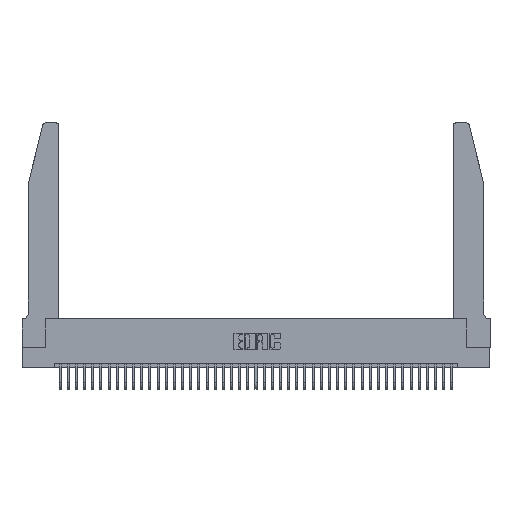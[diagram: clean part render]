
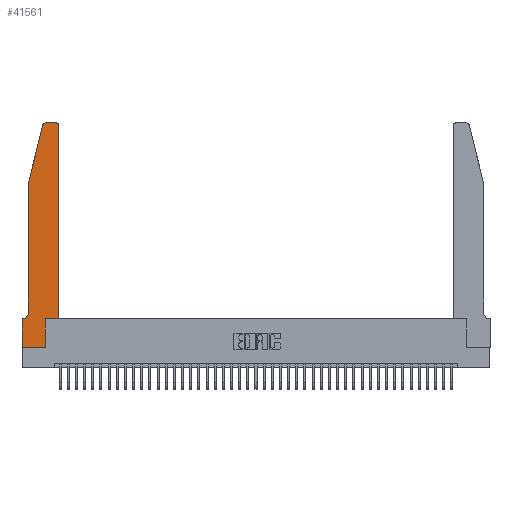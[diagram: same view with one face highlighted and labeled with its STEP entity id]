
A CAD part, top view. The second image highlights one B-rep face of the part: STEP entity #41561.
In plain terms, the highlighted planar face has unit normal (0, 0, 1).
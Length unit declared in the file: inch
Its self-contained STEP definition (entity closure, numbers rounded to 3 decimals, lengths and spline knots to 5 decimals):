
#1439 = CARTESIAN_POINT ( 'NONE',  ( 0.0055, 0.42, 0.37 ) ) ;
#2660 = VERTEX_POINT ( 'NONE', #24972 ) ;
#2988 = LINE ( 'NONE', #31300, #11111 ) ;
#3441 = CIRCLE ( 'NONE', #13869, 0.03 ) ;
#4783 = VERTEX_POINT ( 'NONE', #22623 ) ;
#4931 = DIRECTION ( 'NONE',  ( -1., 0., 0. ) ) ;
#5466 = DIRECTION ( 'NONE',  ( 1., 0., 0. ) ) ;
#5712 = VERTEX_POINT ( 'NONE', #22765 ) ;
#5819 = DIRECTION ( 'NONE',  ( -1., 0., 0. ) ) ;
#6083 = EDGE_CURVE ( 'NONE', #2660, #15268, #40736, .T. ) ;
#6863 = CARTESIAN_POINT ( 'NONE',  ( 0.0755, 0.42, 0.37 ) ) ;
#6955 = EDGE_CURVE ( 'NONE', #35982, #40524, #16182, .T. ) ;
#7196 = EDGE_LOOP ( 'NONE', ( #37225, #29866, #19095, #36758, #37483, #36531, #28214, #31045, #24178, #24218, #27506, #36055 ) ) ;
#9050 = LINE ( 'NONE', #19337, #26089 ) ;
#10390 = CARTESIAN_POINT ( 'NONE',  ( 0.0055, 0.35, 0.37 ) ) ;
#10664 = EDGE_CURVE ( 'NONE', #40524, #4783, #24814, .T. ) ;
#10787 = AXIS2_PLACEMENT_3D ( 'NONE', #39410, #36333, #16208 ) ;
#10838 = VERTEX_POINT ( 'NONE', #14227 ) ;
#11111 = VECTOR ( 'NONE', #28076, 39.37008 ) ;
#11999 = FACE_OUTER_BOUND ( 'NONE', #7196, .T. ) ;
#12035 = LINE ( 'NONE', #25450, #37867 ) ;
#12830 = VECTOR ( 'NONE', #5819, 39.37008 ) ;
#13761 = EDGE_CURVE ( 'NONE', #25990, #34510, #20774, .T. ) ;
#13869 = AXIS2_PLACEMENT_3D ( 'NONE', #35233, #15091, #38585 ) ;
#13967 = CARTESIAN_POINT ( 'NONE',  ( 0., 0.35, 0.37 ) ) ;
#13970 = VERTEX_POINT ( 'NONE', #6863 ) ;
#14227 = CARTESIAN_POINT ( 'NONE',  ( 0.25487, 2.72718, 0.37 ) ) ;
#14809 = AXIS2_PLACEMENT_3D ( 'NONE', #1439, #25410, #4931 ) ;
#15091 = DIRECTION ( 'NONE',  ( 0., 0., 1. ) ) ;
#15139 = VERTEX_POINT ( 'NONE', #42576 ) ;
#15147 = EDGE_CURVE ( 'NONE', #4783, #28723, #9050, .T. ) ;
#15268 = VERTEX_POINT ( 'NONE', #16577 ) ;
#15402 = AXIS2_PLACEMENT_3D ( 'NONE', #17854, #41301, #21235 ) ;
#15629 = EDGE_CURVE ( 'NONE', #5712, #10838, #3441, .T. ) ;
#15688 = LINE ( 'NONE', #20972, #32510 ) ;
#16182 = LINE ( 'NONE', #25915, #33009 ) ;
#16208 = DIRECTION ( 'NONE',  ( 1., 0., 0. ) ) ;
#16577 = CARTESIAN_POINT ( 'NONE',  ( 0.4205, 2.75, 0.37 ) ) ;
#17854 = CARTESIAN_POINT ( 'NONE',  ( 0.4205, 2.72, 0.37 ) ) ;
#18357 = CIRCLE ( 'NONE', #14809, 0.07 ) ;
#19095 = ORIENTED_EDGE ( 'NONE', *, *, #28582, .T. ) ;
#19337 = CARTESIAN_POINT ( 'NONE',  ( 0.4505, 0.35, 0.37 ) ) ;
#19464 = PLANE ( 'NONE',  #10787 ) ;
#19809 = EDGE_CURVE ( 'NONE', #15139, #13970, #20730, .T. ) ;
#20730 = LINE ( 'NONE', #32227, #37535 ) ;
#20774 = LINE ( 'NONE', #29625, #12830 ) ;
#20972 = CARTESIAN_POINT ( 'NONE',  ( 0.0755, 2., 0.37 ) ) ;
#21235 = DIRECTION ( 'NONE',  ( 1., 0., 0. ) ) ;
#21763 = EDGE_CURVE ( 'NONE', #15268, #5712, #23233, .T. ) ;
#22623 = CARTESIAN_POINT ( 'NONE',  ( 0.2865, 0.35, 0.37 ) ) ;
#22765 = CARTESIAN_POINT ( 'NONE',  ( 0.284, 2.75, 0.37 ) ) ;
#23233 = LINE ( 'NONE', #28748, #31067 ) ;
#23754 = VECTOR ( 'NONE', #37024, 39.37008 ) ;
#24178 = ORIENTED_EDGE ( 'NONE', *, *, #10664, .T. ) ;
#24218 = ORIENTED_EDGE ( 'NONE', *, *, #15147, .T. ) ;
#24377 = DIRECTION ( 'NONE',  ( -0.239, -0.971, 0. ) ) ;
#24814 = LINE ( 'NONE', #33669, #23754 ) ;
#24972 = CARTESIAN_POINT ( 'NONE',  ( 0.4505, 2.72, 0.37 ) ) ;
#25410 = DIRECTION ( 'NONE',  ( 0., 0., -1. ) ) ;
#25450 = CARTESIAN_POINT ( 'NONE',  ( 0.4505, 0.35, 0.37 ) ) ;
#25915 = CARTESIAN_POINT ( 'NONE',  ( 0., 0., 0.37 ) ) ;
#25990 = VERTEX_POINT ( 'NONE', #10390 ) ;
#26089 = VECTOR ( 'NONE', #32693, 39.37008 ) ;
#26416 = EDGE_CURVE ( 'NONE', #28723, #2660, #12035, .T. ) ;
#27506 = ORIENTED_EDGE ( 'NONE', *, *, #26416, .T. ) ;
#28076 = DIRECTION ( 'NONE',  ( 0., -1., 0. ) ) ;
#28214 = ORIENTED_EDGE ( 'NONE', *, *, #39226, .T. ) ;
#28321 = CARTESIAN_POINT ( 'NONE',  ( 0.4505, 0.35, 0.37 ) ) ;
#28582 = EDGE_CURVE ( 'NONE', #10838, #15139, #15688, .T. ) ;
#28723 = VERTEX_POINT ( 'NONE', #28321 ) ;
#28748 = CARTESIAN_POINT ( 'NONE',  ( 0.2605, 2.75, 0.37 ) ) ;
#28899 = DIRECTION ( 'NONE',  ( -1., 0., 0. ) ) ;
#29152 = CARTESIAN_POINT ( 'NONE',  ( 0.2865, 0., 0.37 ) ) ;
#29625 = CARTESIAN_POINT ( 'NONE',  ( 0.0755, 0.35, 0.37 ) ) ;
#29866 = ORIENTED_EDGE ( 'NONE', *, *, #15629, .T. ) ;
#30908 = CARTESIAN_POINT ( 'NONE',  ( 0., 0., 0.37 ) ) ;
#31045 = ORIENTED_EDGE ( 'NONE', *, *, #6955, .T. ) ;
#31067 = VECTOR ( 'NONE', #28899, 39.37008 ) ;
#31300 = CARTESIAN_POINT ( 'NONE',  ( 0., 0., 0.37 ) ) ;
#32227 = CARTESIAN_POINT ( 'NONE',  ( 0.0755, 2., 0.37 ) ) ;
#32510 = VECTOR ( 'NONE', #24377, 39.37008 ) ;
#32693 = DIRECTION ( 'NONE',  ( 1., 0., 0. ) ) ;
#33009 = VECTOR ( 'NONE', #5466, 39.37008 ) ;
#33669 = CARTESIAN_POINT ( 'NONE',  ( 0.2865, 0.35, 0.37 ) ) ;
#34510 = VERTEX_POINT ( 'NONE', #13967 ) ;
#35233 = CARTESIAN_POINT ( 'NONE',  ( 0.284, 2.72, 0.37 ) ) ;
#35596 = DIRECTION ( 'NONE',  ( 0., -1., 0. ) ) ;
#35982 = VERTEX_POINT ( 'NONE', #30908 ) ;
#36055 = ORIENTED_EDGE ( 'NONE', *, *, #6083, .T. ) ;
#36333 = DIRECTION ( 'NONE',  ( 0., 0., 1. ) ) ;
#36531 = ORIENTED_EDGE ( 'NONE', *, *, #13761, .T. ) ;
#36758 = ORIENTED_EDGE ( 'NONE', *, *, #19809, .T. ) ;
#37024 = DIRECTION ( 'NONE',  ( 0., 1., 0. ) ) ;
#37225 = ORIENTED_EDGE ( 'NONE', *, *, #21763, .T. ) ;
#37483 = ORIENTED_EDGE ( 'NONE', *, *, #38068, .T. ) ;
#37535 = VECTOR ( 'NONE', #35596, 39.37008 ) ;
#37867 = VECTOR ( 'NONE', #42126, 39.37008 ) ;
#38068 = EDGE_CURVE ( 'NONE', #13970, #25990, #18357, .T. ) ;
#38585 = DIRECTION ( 'NONE',  ( 1., 0., 0. ) ) ;
#39226 = EDGE_CURVE ( 'NONE', #34510, #35982, #2988, .T. ) ;
#39410 = CARTESIAN_POINT ( 'NONE',  ( 0., 0.35, 0.37 ) ) ;
#40524 = VERTEX_POINT ( 'NONE', #29152 ) ;
#40736 = CIRCLE ( 'NONE', #15402, 0.03 ) ;
#41301 = DIRECTION ( 'NONE',  ( 0., 0., 1. ) ) ;
#41561 = ADVANCED_FACE ( 'NONE', ( #11999 ), #19464, .T. ) ;
#42126 = DIRECTION ( 'NONE',  ( 0., 1., 0. ) ) ;
#42576 = CARTESIAN_POINT ( 'NONE',  ( 0.0755, 2., 0.37 ) ) ;
